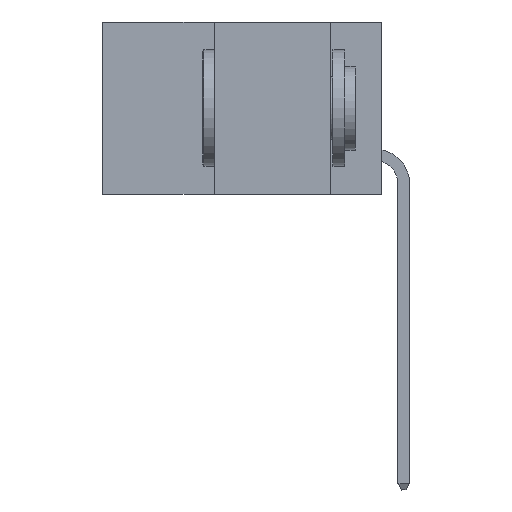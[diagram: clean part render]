
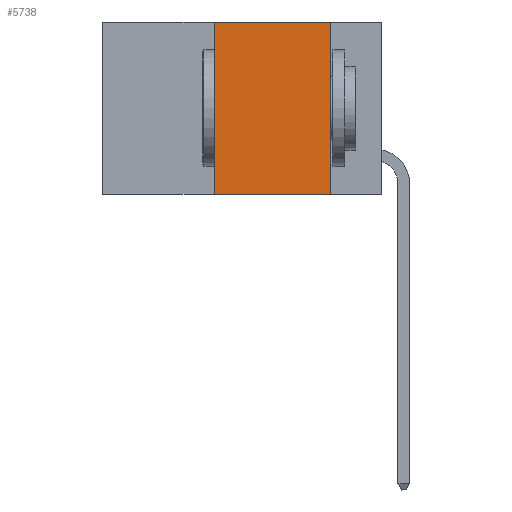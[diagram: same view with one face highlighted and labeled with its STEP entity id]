
A CAD part, left-side view. The second image highlights one B-rep face of the part: STEP entity #5738.
In plain terms, the highlighted planar face has unit normal (-1, 0, 0).
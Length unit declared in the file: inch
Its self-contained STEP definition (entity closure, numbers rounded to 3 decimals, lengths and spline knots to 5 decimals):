
#221 = DIRECTION ( 'NONE',  ( 0., -1., 0. ) ) ;
#288 = VECTOR ( 'NONE', #221, 39.37008 ) ;
#729 = EDGE_CURVE ( 'NONE', #19589, #3158, #16317, .T. ) ;
#764 = CARTESIAN_POINT ( 'NONE',  ( 0., 0.36, 0. ) ) ;
#2602 = DIRECTION ( 'NONE',  ( 0., 0., -1. ) ) ;
#2986 = CARTESIAN_POINT ( 'NONE',  ( 0., 0.11, 0. ) ) ;
#3158 = VERTEX_POINT ( 'NONE', #22765 ) ;
#4281 = EDGE_CURVE ( 'NONE', #19374, #13776, #10754, .T. ) ;
#4475 = VECTOR ( 'NONE', #22352, 39.37008 ) ;
#4643 = EDGE_CURVE ( 'NONE', #13776, #3158, #24430, .T. ) ;
#5738 = ADVANCED_FACE ( 'NONE', ( #9245 ), #14716, .F. ) ;
#6240 = CARTESIAN_POINT ( 'NONE',  ( 0., 0.6, -0.37 ) ) ;
#7949 = ORIENTED_EDGE ( 'NONE', *, *, #4643, .F. ) ;
#8399 = CARTESIAN_POINT ( 'NONE',  ( 0., 0.6, 0. ) ) ;
#9245 = FACE_OUTER_BOUND ( 'NONE', #19697, .T. ) ;
#9361 = CARTESIAN_POINT ( 'NONE',  ( 0., 0.11, 0. ) ) ;
#10754 = LINE ( 'NONE', #24466, #288 ) ;
#12325 = VECTOR ( 'NONE', #19260, 39.37008 ) ;
#12385 = AXIS2_PLACEMENT_3D ( 'NONE', #8399, #20873, #2602 ) ;
#12845 = VECTOR ( 'NONE', #24421, 39.37008 ) ;
#13776 = VERTEX_POINT ( 'NONE', #9361 ) ;
#14716 = PLANE ( 'NONE',  #12385 ) ;
#16317 = LINE ( 'NONE', #6240, #12845 ) ;
#16442 = ORIENTED_EDGE ( 'NONE', *, *, #4281, .F. ) ;
#17537 = CARTESIAN_POINT ( 'NONE',  ( 0., 0.36, -0.37 ) ) ;
#18116 = LINE ( 'NONE', #18138, #4475 ) ;
#18138 = CARTESIAN_POINT ( 'NONE',  ( 0., 0.36, 0. ) ) ;
#19260 = DIRECTION ( 'NONE',  ( 0., 0., -1. ) ) ;
#19374 = VERTEX_POINT ( 'NONE', #764 ) ;
#19589 = VERTEX_POINT ( 'NONE', #17537 ) ;
#19697 = EDGE_LOOP ( 'NONE', ( #7949, #16442, #22880, #21110 ) ) ;
#19787 = EDGE_CURVE ( 'NONE', #19589, #19374, #18116, .T. ) ;
#20873 = DIRECTION ( 'NONE',  ( 1., 0., 0. ) ) ;
#21110 = ORIENTED_EDGE ( 'NONE', *, *, #729, .T. ) ;
#22352 = DIRECTION ( 'NONE',  ( 0., 0., 1. ) ) ;
#22765 = CARTESIAN_POINT ( 'NONE',  ( 0., 0.11, -0.37 ) ) ;
#22880 = ORIENTED_EDGE ( 'NONE', *, *, #19787, .F. ) ;
#24421 = DIRECTION ( 'NONE',  ( 0., -1., 0. ) ) ;
#24430 = LINE ( 'NONE', #2986, #12325 ) ;
#24466 = CARTESIAN_POINT ( 'NONE',  ( 0., 0.6, 0. ) ) ;
